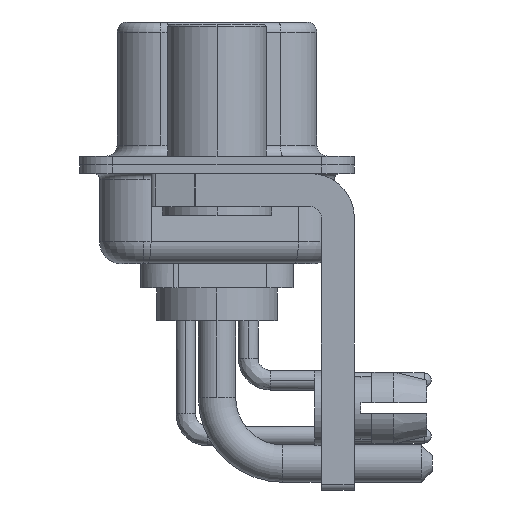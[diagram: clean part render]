
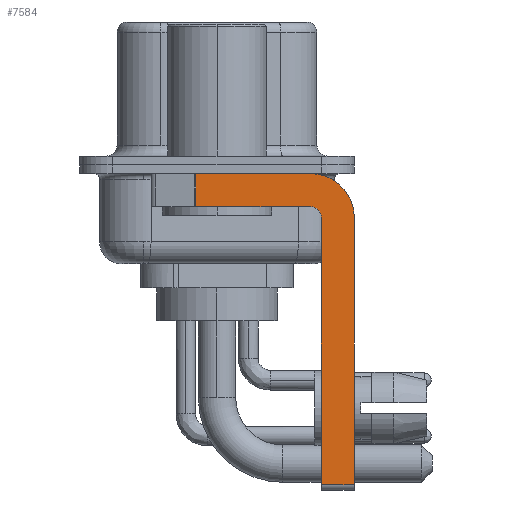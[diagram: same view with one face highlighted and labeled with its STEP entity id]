
A CAD part, left-side view. The second image highlights one B-rep face of the part: STEP entity #7584.
In plain terms, the highlighted planar face has unit normal (-1, 0, 0).
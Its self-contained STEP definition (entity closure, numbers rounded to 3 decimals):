
#9 = AXIS2_PLACEMENT_3D ( 'NONE', #14364, #13332, #20930 ) ;
#452 = VERTEX_POINT ( 'NONE', #8615 ) ;
#614 = LINE ( 'NONE', #15495, #10632 ) ;
#663 = CARTESIAN_POINT ( 'NONE',  ( -2.9, -4.25, -0.4 ) ) ;
#842 = DIRECTION ( 'NONE',  ( 0., -1., 0. ) ) ;
#1799 = CARTESIAN_POINT ( 'NONE',  ( -2.9, 0.978, -1.9 ) ) ;
#1976 = ORIENTED_EDGE ( 'NONE', *, *, #15217, .F. ) ;
#2361 = ORIENTED_EDGE ( 'NONE', *, *, #9093, .F. ) ;
#2477 = VECTOR ( 'NONE', #842, 1000. ) ;
#2549 = CARTESIAN_POINT ( 'NONE',  ( -2.9, -4.75, -14.55 ) ) ;
#2572 = EDGE_CURVE ( 'NONE', #16025, #25925, #614, .T. ) ;
#3574 = DIRECTION ( 'NONE',  ( 0., 0., -1. ) ) ;
#5361 = VECTOR ( 'NONE', #15521, 1000. ) ;
#5448 = CARTESIAN_POINT ( 'NONE',  ( -2.9, -4.25, -14.55 ) ) ;
#5885 = DIRECTION ( 'NONE',  ( -1., 0., 0. ) ) ;
#6058 = LINE ( 'NONE', #16132, #16139 ) ;
#6665 = ORIENTED_EDGE ( 'NONE', *, *, #30579, .T. ) ;
#7339 = ORIENTED_EDGE ( 'NONE', *, *, #2572, .F. ) ;
#7584 = ADVANCED_FACE ( 'NONE', ( #29196 ), #26718, .F. ) ;
#7779 = LINE ( 'NONE', #5448, #5361 ) ;
#8615 = CARTESIAN_POINT ( 'NONE',  ( -2.9, 0.978, -0.4 ) ) ;
#9093 = EDGE_CURVE ( 'NONE', #32517, #16025, #19361, .T. ) ;
#9307 = CARTESIAN_POINT ( 'NONE',  ( -2.9, -4.25, -1.9 ) ) ;
#10632 = VECTOR ( 'NONE', #30378, 1000. ) ;
#12637 = CARTESIAN_POINT ( 'NONE',  ( -2.9, -4.75, -14.8 ) ) ;
#13320 = EDGE_CURVE ( 'NONE', #452, #25925, #30308, .T. ) ;
#13332 = DIRECTION ( 'NONE',  ( 1., 0., 0. ) ) ;
#13809 = DIRECTION ( 'NONE',  ( 0., 0., 1. ) ) ;
#13904 = CARTESIAN_POINT ( 'NONE',  ( -2.9, -6.25, -14.55 ) ) ;
#14171 = CARTESIAN_POINT ( 'NONE',  ( -2.9, -4.25, -2.4 ) ) ;
#14364 = CARTESIAN_POINT ( 'NONE',  ( -2.9, -4.25, -2.4 ) ) ;
#14384 = EDGE_CURVE ( 'NONE', #30733, #20155, #6058, .T. ) ;
#15217 = EDGE_CURVE ( 'NONE', #452, #21874, #15888, .T. ) ;
#15495 = CARTESIAN_POINT ( 'NONE',  ( -2.9, -4.25, -1.9 ) ) ;
#15521 = DIRECTION ( 'NONE',  ( 0., -1., 0. ) ) ;
#15774 = VECTOR ( 'NONE', #27669, 1000. ) ;
#15888 = LINE ( 'NONE', #23974, #2477 ) ;
#16025 = VERTEX_POINT ( 'NONE', #9307 ) ;
#16132 = CARTESIAN_POINT ( 'NONE',  ( -2.9, -6.25, -2.4 ) ) ;
#16139 = VECTOR ( 'NONE', #3574, 1000. ) ;
#17123 = LINE ( 'NONE', #12637, #15774 ) ;
#17746 = CARTESIAN_POINT ( 'NONE',  ( -2.9, 0.978, -1.9 ) ) ;
#19361 = CIRCLE ( 'NONE', #25135, 0.5 ) ;
#20155 = VERTEX_POINT ( 'NONE', #13904 ) ;
#20915 = VECTOR ( 'NONE', #25492, 1000. ) ;
#20930 = DIRECTION ( 'NONE',  ( 0., 0., -1. ) ) ;
#21078 = CARTESIAN_POINT ( 'NONE',  ( -2.9, -4.25, -2.4 ) ) ;
#21271 = CARTESIAN_POINT ( 'NONE',  ( -2.9, -4.75, -2.4 ) ) ;
#21634 = CARTESIAN_POINT ( 'NONE',  ( -2.9, -6.25, -2.4 ) ) ;
#21874 = VERTEX_POINT ( 'NONE', #663 ) ;
#23175 = ORIENTED_EDGE ( 'NONE', *, *, #28233, .F. ) ;
#23230 = ORIENTED_EDGE ( 'NONE', *, *, #31032, .F. ) ;
#23294 = VERTEX_POINT ( 'NONE', #2549 ) ;
#23974 = CARTESIAN_POINT ( 'NONE',  ( -2.9, 3., -0.4 ) ) ;
#25135 = AXIS2_PLACEMENT_3D ( 'NONE', #21078, #5885, #13809 ) ;
#25492 = DIRECTION ( 'NONE',  ( 0., 0., -1. ) ) ;
#25925 = VERTEX_POINT ( 'NONE', #1799 ) ;
#26718 = PLANE ( 'NONE',  #30224 ) ;
#26882 = DIRECTION ( 'NONE',  ( 1., 0., 0. ) ) ;
#27669 = DIRECTION ( 'NONE',  ( 0., 0., 1. ) ) ;
#28233 = EDGE_CURVE ( 'NONE', #23294, #32517, #17123, .T. ) ;
#28504 = CIRCLE ( 'NONE', #9, 2. ) ;
#29196 = FACE_OUTER_BOUND ( 'NONE', #30240, .T. ) ;
#29926 = ORIENTED_EDGE ( 'NONE', *, *, #13320, .T. ) ;
#30224 = AXIS2_PLACEMENT_3D ( 'NONE', #14171, #26882, #32178 ) ;
#30240 = EDGE_LOOP ( 'NONE', ( #1976, #29926, #7339, #2361, #23175, #6665, #31870, #23230 ) ) ;
#30308 = LINE ( 'NONE', #17746, #20915 ) ;
#30378 = DIRECTION ( 'NONE',  ( 0., 1., 0. ) ) ;
#30579 = EDGE_CURVE ( 'NONE', #23294, #20155, #7779, .T. ) ;
#30733 = VERTEX_POINT ( 'NONE', #21634 ) ;
#31032 = EDGE_CURVE ( 'NONE', #21874, #30733, #28504, .T. ) ;
#31870 = ORIENTED_EDGE ( 'NONE', *, *, #14384, .F. ) ;
#32178 = DIRECTION ( 'NONE',  ( 0., 0., -1. ) ) ;
#32517 = VERTEX_POINT ( 'NONE', #21271 ) ;
